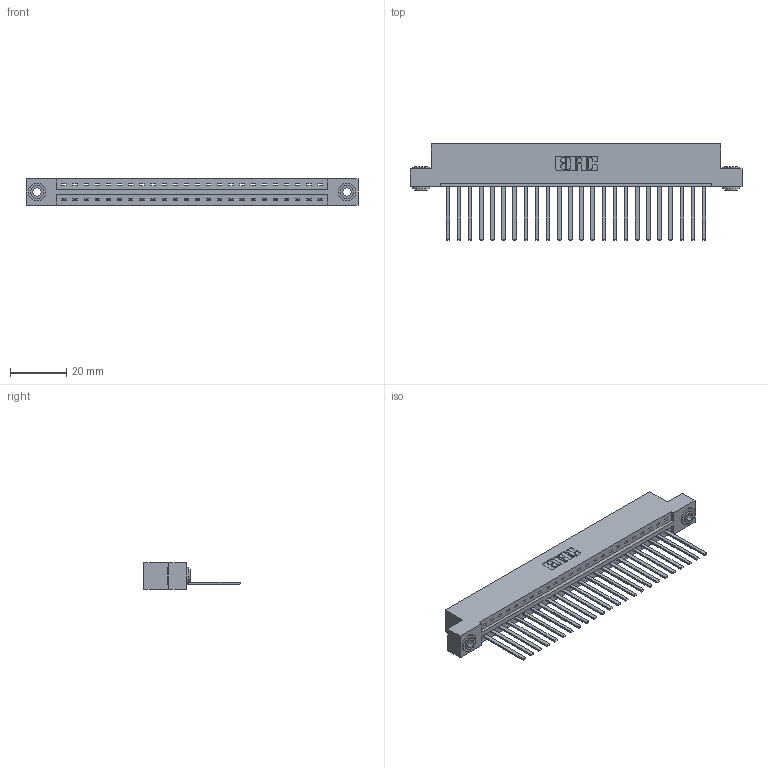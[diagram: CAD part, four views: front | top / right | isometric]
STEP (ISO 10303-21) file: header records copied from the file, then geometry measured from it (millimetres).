
FILE_DESCRIPTION (( 'STEP AP203' ), '1' );
FILE_NAME ('337-024-544-103.STEP', '2019-09-30T16:05:10', ( '' ), ( '' ), 'SwSTEP 2.0', 'SolidWorks 2016', '' );
FILE_SCHEMA (( 'CONFIG_CONTROL_DESIGN' ));
Length unit declared in the file: inch
Products named in the file (4): 345-292-001_345-293-144; 345-250-002_345-250-002-102; 337 Part_Flush Mounting Lugs - 0.156 Dia-TH; 337-024-544-103
Assembly tree (27 placements, depth 2):
  337-024-544-103
    337 Part_Flush Mounting Lugs - 0.156 Dia-TH
    345-292-001_345-293-144  x24
    345-250-002_345-250-002-102  x2
Bounding box: 118.11 x 34.3 x 9.4 mm (x, y, z)
Volume: 12347.6 mm3; surface area: 13806.6 mm2
Topology: 27 solids, 27 shells, 1496 faces, 4467 edges, 2942 vertices
Faces by surface type: plane 1088, cylinder 400, cone 8
Entity records: 20634 total; most frequent: CARTESIAN_POINT 3569, ORIENTED_EDGE 3522, DIRECTION 3071, EDGE_CURVE 1761, LINE 1613, VECTOR 1613, VERTEX_POINT 1170, AXIS2_PLACEMENT_3D 729
